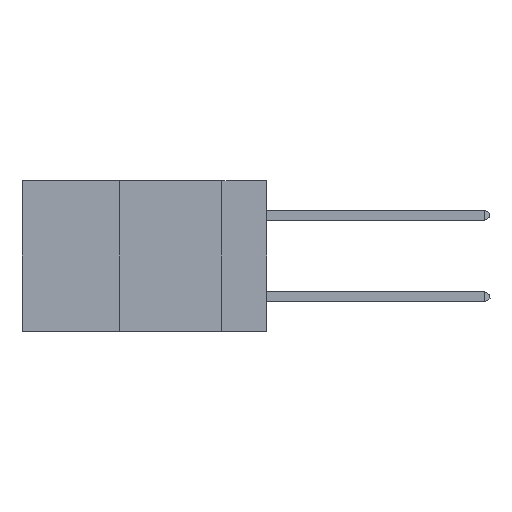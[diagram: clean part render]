
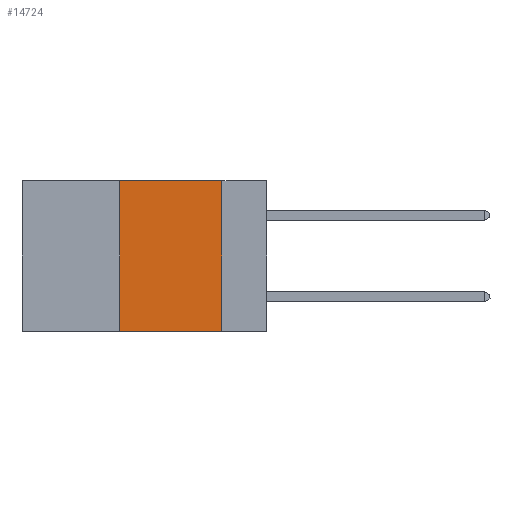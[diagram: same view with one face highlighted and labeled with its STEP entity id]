
A CAD part, left-side view. The second image highlights one B-rep face of the part: STEP entity #14724.
In plain terms, the highlighted planar face has unit normal (-1, 0, 0).
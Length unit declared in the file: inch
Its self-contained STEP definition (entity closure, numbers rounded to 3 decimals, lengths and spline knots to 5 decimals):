
#185 = VERTEX_POINT ( 'NONE', #9399 ) ;
#845 = AXIS2_PLACEMENT_3D ( 'NONE', #1489, #13210, #4504 ) ;
#1489 = CARTESIAN_POINT ( 'NONE',  ( 0., 0.6, 0. ) ) ;
#1526 = CARTESIAN_POINT ( 'NONE',  ( 0., 0.6, -0.37 ) ) ;
#1896 = VECTOR ( 'NONE', #8010, 39.37008 ) ;
#2528 = VECTOR ( 'NONE', #5517, 39.37008 ) ;
#2851 = VERTEX_POINT ( 'NONE', #10887 ) ;
#2994 = ORIENTED_EDGE ( 'NONE', *, *, #18349, .F. ) ;
#3756 = LINE ( 'NONE', #11455, #18635 ) ;
#4218 = FACE_OUTER_BOUND ( 'NONE', #15173, .T. ) ;
#4504 = DIRECTION ( 'NONE',  ( 0., 0., -1. ) ) ;
#5517 = DIRECTION ( 'NONE',  ( 0., -1., 0. ) ) ;
#6314 = VERTEX_POINT ( 'NONE', #14081 ) ;
#6441 = EDGE_CURVE ( 'NONE', #6314, #2851, #3756, .T. ) ;
#6529 = CARTESIAN_POINT ( 'NONE',  ( 0., 0.36, 0. ) ) ;
#6960 = LINE ( 'NONE', #9852, #2528 ) ;
#7439 = ORIENTED_EDGE ( 'NONE', *, *, #8587, .T. ) ;
#8010 = DIRECTION ( 'NONE',  ( 0., 0., 1. ) ) ;
#8587 = EDGE_CURVE ( 'NONE', #16302, #2851, #9748, .T. ) ;
#9399 = CARTESIAN_POINT ( 'NONE',  ( 0., 0.36, 0. ) ) ;
#9748 = LINE ( 'NONE', #1526, #14860 ) ;
#9788 = LINE ( 'NONE', #6529, #1896 ) ;
#9852 = CARTESIAN_POINT ( 'NONE',  ( 0., 0.6, 0. ) ) ;
#10406 = DIRECTION ( 'NONE',  ( 0., -1., 0. ) ) ;
#10887 = CARTESIAN_POINT ( 'NONE',  ( 0., 0.11, -0.37 ) ) ;
#11455 = CARTESIAN_POINT ( 'NONE',  ( 0., 0.11, 0. ) ) ;
#11779 = PLANE ( 'NONE',  #845 ) ;
#13210 = DIRECTION ( 'NONE',  ( 1., 0., 0. ) ) ;
#14081 = CARTESIAN_POINT ( 'NONE',  ( 0., 0.11, 0. ) ) ;
#14191 = ORIENTED_EDGE ( 'NONE', *, *, #6441, .F. ) ;
#14724 = ADVANCED_FACE ( 'NONE', ( #4218 ), #11779, .F. ) ;
#14859 = EDGE_CURVE ( 'NONE', #16302, #185, #9788, .T. ) ;
#14860 = VECTOR ( 'NONE', #10406, 39.37008 ) ;
#15173 = EDGE_LOOP ( 'NONE', ( #14191, #2994, #18368, #7439 ) ) ;
#16030 = CARTESIAN_POINT ( 'NONE',  ( 0., 0.36, -0.37 ) ) ;
#16302 = VERTEX_POINT ( 'NONE', #16030 ) ;
#18349 = EDGE_CURVE ( 'NONE', #185, #6314, #6960, .T. ) ;
#18368 = ORIENTED_EDGE ( 'NONE', *, *, #14859, .F. ) ;
#18508 = DIRECTION ( 'NONE',  ( 0., 0., -1. ) ) ;
#18635 = VECTOR ( 'NONE', #18508, 39.37008 ) ;
